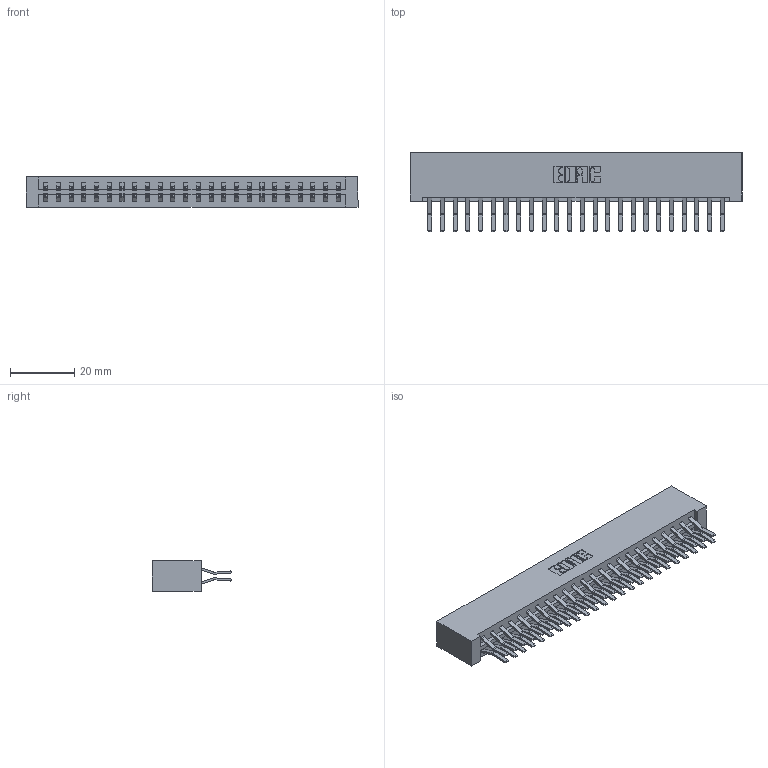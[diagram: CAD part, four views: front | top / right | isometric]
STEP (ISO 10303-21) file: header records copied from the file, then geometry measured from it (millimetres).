
FILE_DESCRIPTION (( 'STEP AP203' ), '1' );
FILE_NAME ('833-048-560-201.STEP', '2020-06-04T16:45:56', ( '' ), ( '' ), 'SwSTEP 2.0', 'SolidWorks 2020', '' );
FILE_SCHEMA (( 'CONFIG_CONTROL_DESIGN' ));
Length unit declared in the file: inch
Products named in the file (3): 345-292-001_560 Tail; 833-048-560-201; 833 Part_Lugless
Assembly tree (49 placements, depth 2):
  833-048-560-201
    833 Part_Lugless
    345-292-001_560 Tail  x48
Bounding box: 103.35 x 24.78 x 9.4 mm (x, y, z)
Volume: 11330.2 mm3; surface area: 14123.6 mm2
Topology: 49 solids, 49 shells, 2698 faces, 8015 edges, 5278 vertices
Faces by surface type: plane 1794, cylinder 904
Entity records: 17579 total; most frequent: CARTESIAN_POINT 2934, ORIENTED_EDGE 2870, DIRECTION 2535, EDGE_CURVE 1435, VECTOR 1311, LINE 1311, VERTEX_POINT 954, AXIS2_PLACEMENT_3D 612
